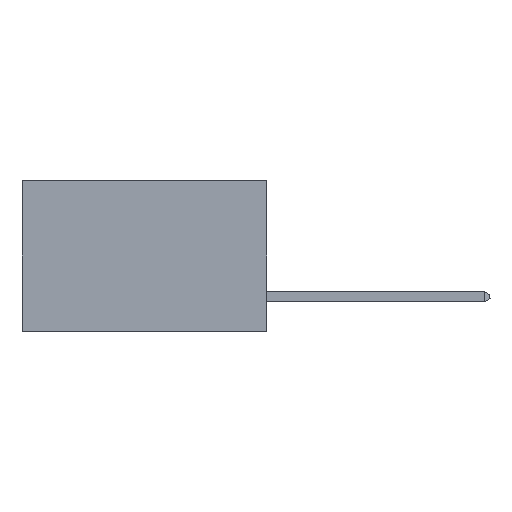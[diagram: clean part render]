
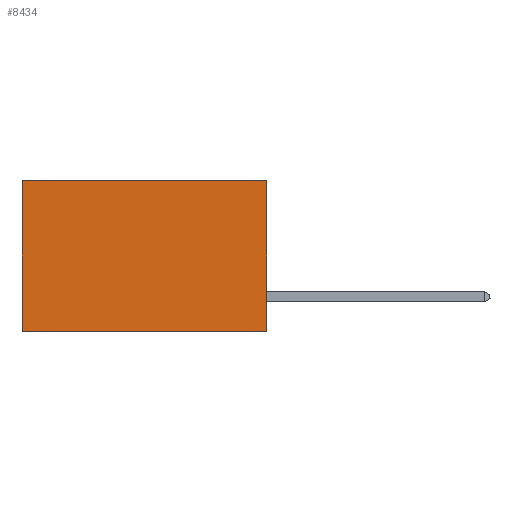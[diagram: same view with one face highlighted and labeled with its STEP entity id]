
A CAD part, left-side view. The second image highlights one B-rep face of the part: STEP entity #8434.
In plain terms, the highlighted planar face has unit normal (-1, 0, 0).
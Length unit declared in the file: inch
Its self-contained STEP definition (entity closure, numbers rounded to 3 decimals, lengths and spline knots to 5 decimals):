
#2070 = DIRECTION ( 'NONE',  ( 0., 0., -1. ) ) ;
#2337 = AXIS2_PLACEMENT_3D ( 'NONE', #4566, #7572, #3229 ) ;
#2536 = DIRECTION ( 'NONE',  ( 0., 0., -1. ) ) ;
#3012 = VERTEX_POINT ( 'NONE', #17219 ) ;
#3229 = DIRECTION ( 'NONE',  ( 0., 0., -1. ) ) ;
#3392 = VECTOR ( 'NONE', #2070, 39.37008 ) ;
#4140 = LINE ( 'NONE', #17666, #16317 ) ;
#4216 = ORIENTED_EDGE ( 'NONE', *, *, #8666, .T. ) ;
#4524 = FACE_OUTER_BOUND ( 'NONE', #17282, .T. ) ;
#4566 = CARTESIAN_POINT ( 'NONE',  ( 0.2875, 0., 0. ) ) ;
#6423 = CARTESIAN_POINT ( 'NONE',  ( 0.2875, 0., 0. ) ) ;
#7516 = DIRECTION ( 'NONE',  ( 0., 1., 0. ) ) ;
#7528 = LINE ( 'NONE', #18694, #15752 ) ;
#7572 = DIRECTION ( 'NONE',  ( 1., 0., 0. ) ) ;
#7921 = EDGE_CURVE ( 'NONE', #14144, #15567, #11652, .T. ) ;
#8434 = ADVANCED_FACE ( 'NONE', ( #4524 ), #10372, .F. ) ;
#8666 = EDGE_CURVE ( 'NONE', #14144, #3012, #18512, .T. ) ;
#8734 = CARTESIAN_POINT ( 'NONE',  ( 0.2875, 0., 0. ) ) ;
#9216 = ORIENTED_EDGE ( 'NONE', *, *, #12920, .F. ) ;
#10372 = PLANE ( 'NONE',  #2337 ) ;
#11652 = LINE ( 'NONE', #6423, #3392 ) ;
#11851 = CARTESIAN_POINT ( 'NONE',  ( 0.2875, 0.6, -0.37 ) ) ;
#11999 = ORIENTED_EDGE ( 'NONE', *, *, #7921, .F. ) ;
#12858 = CARTESIAN_POINT ( 'NONE',  ( 0.2875, 0., -0.37 ) ) ;
#12920 = EDGE_CURVE ( 'NONE', #15567, #17982, #4140, .T. ) ;
#14144 = VERTEX_POINT ( 'NONE', #8734 ) ;
#14637 = VECTOR ( 'NONE', #15581, 39.37008 ) ;
#14924 = EDGE_CURVE ( 'NONE', #3012, #17982, #7528, .T. ) ;
#15567 = VERTEX_POINT ( 'NONE', #12858 ) ;
#15581 = DIRECTION ( 'NONE',  ( 0., 1., 0. ) ) ;
#15752 = VECTOR ( 'NONE', #2536, 39.37008 ) ;
#16317 = VECTOR ( 'NONE', #7516, 39.37008 ) ;
#16736 = ORIENTED_EDGE ( 'NONE', *, *, #14924, .T. ) ;
#17059 = CARTESIAN_POINT ( 'NONE',  ( 0.2875, 0., 0. ) ) ;
#17219 = CARTESIAN_POINT ( 'NONE',  ( 0.2875, 0.6, 0. ) ) ;
#17282 = EDGE_LOOP ( 'NONE', ( #16736, #9216, #11999, #4216 ) ) ;
#17666 = CARTESIAN_POINT ( 'NONE',  ( 0.2875, 0., -0.37 ) ) ;
#17982 = VERTEX_POINT ( 'NONE', #11851 ) ;
#18512 = LINE ( 'NONE', #17059, #14637 ) ;
#18694 = CARTESIAN_POINT ( 'NONE',  ( 0.2875, 0.6, 0. ) ) ;
